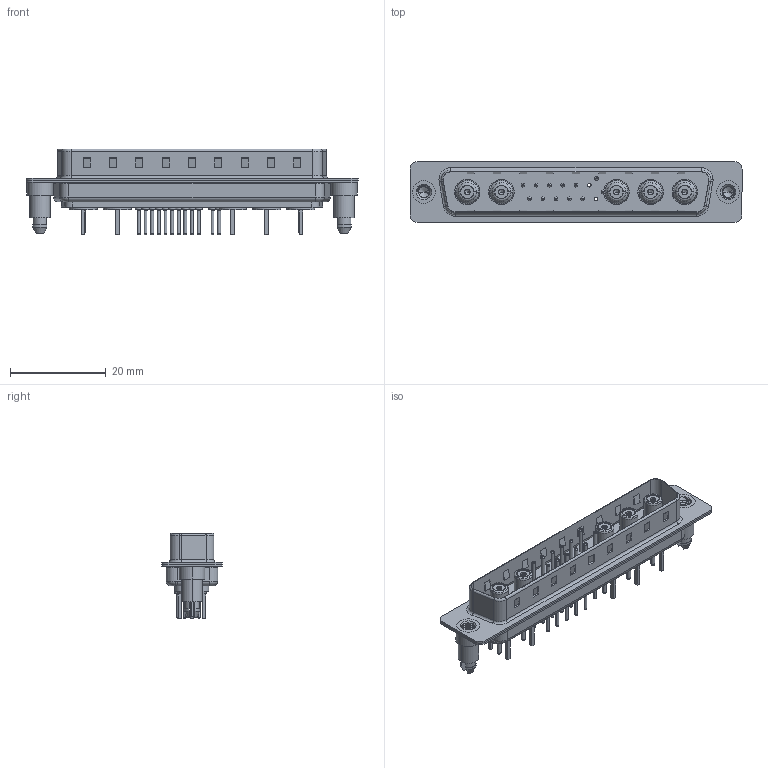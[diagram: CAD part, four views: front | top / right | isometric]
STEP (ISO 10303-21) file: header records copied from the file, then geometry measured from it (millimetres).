
FILE_DESCRIPTION (( 'STEP AP203' ), '1' );
FILE_NAME ('627-17W5224-5ND.STEP', '2019-05-29T03:39:46', ( '' ), ( '' ), 'SwSTEP 2.0', 'SolidWorks 2016', '' );
FILE_SCHEMA (( 'CONFIG_CONTROL_DESIGN' ));
Length unit declared in the file: millimetre
Products named in the file (14): Locking Collar; Socket_Str; 627Combo Housing_17W5; Co-Ax Jack Assy_S; 627Combo Shell Rear_37 Contacts; 627Combo Threaded Boardlock_5; 627Combo Shell Front_37 Contacts; 627Combo Contact Row 1_24; 627Combo Threaded Boardlock_D; 627Combo Contact Row 2_24; Co-Ax Jack_Straight PC Tail; 627-17W5224-5ND; Insulator Socket; Insulator Socket 2
Assembly tree (27 placements, depth 3):
  627-17W5224-5ND
    627Combo Housing_17W5
    627Combo Shell Rear_37 Contacts
    627Combo Shell Front_37 Contacts
    627Combo Threaded Boardlock_D
    Co-Ax Jack Assy_S  x5
      Co-Ax Jack_Straight PC Tail
      Insulator Socket
      Insulator Socket 2
      Locking Collar
      Socket_Str
    627Combo Threaded Boardlock_5
    627Combo Contact Row 1_24  x6
    627Combo Contact Row 2_24  x6
Bounding box: 69.3 x 12.6 x 17.9 mm (x, y, z)
Volume: 4009.5 mm3; surface area: 11462.3 mm2
Topology: 42 solids, 42 shells, 1469 faces, 3342 edges, 2072 vertices
Faces by surface type: cylinder 584, plane 538, torus 262, cone 58, bspline 17, sphere 10
Entity records: 27893 total; most frequent: CARTESIAN_POINT 7894, DIRECTION 3968, ORIENTED_EDGE 3648, EDGE_CURVE 1824, AXIS2_PLACEMENT_3D 1516, VERTEX_POINT 1160, VECTOR 936, LINE 936
